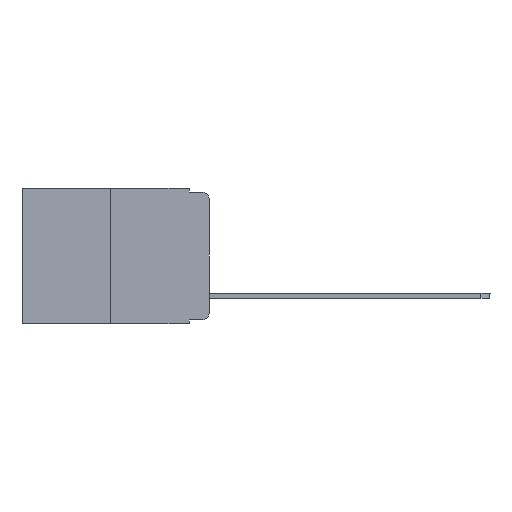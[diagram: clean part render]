
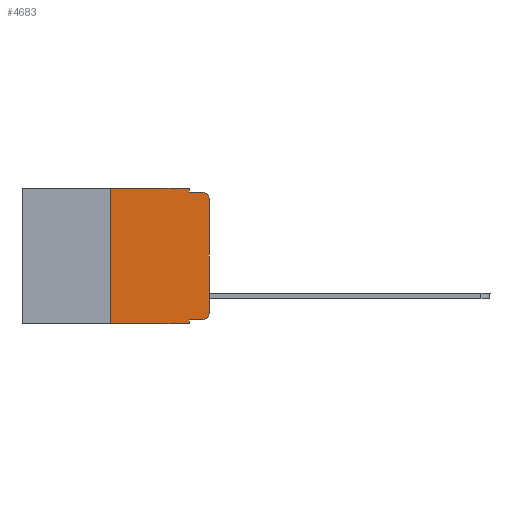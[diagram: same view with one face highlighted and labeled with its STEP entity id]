
A CAD part, left-side view. The second image highlights one B-rep face of the part: STEP entity #4683.
In plain terms, the highlighted planar face has unit normal (-1, 0, 0).
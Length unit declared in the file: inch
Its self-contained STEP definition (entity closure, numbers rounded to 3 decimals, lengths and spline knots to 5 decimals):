
#188 = CARTESIAN_POINT ( 'NONE',  ( 0., 0., -0.03 ) ) ;
#470 = EDGE_CURVE ( 'NONE', #12312, #9007, #893, .T. ) ;
#848 = DIRECTION ( 'NONE',  ( 0., 0., -1. ) ) ;
#893 = LINE ( 'NONE', #14707, #12993 ) ;
#906 = DIRECTION ( 'NONE',  ( 0., 0., -1. ) ) ;
#1216 = VERTEX_POINT ( 'NONE', #9771 ) ;
#1323 = EDGE_CURVE ( 'NONE', #9047, #8708, #15082, .T. ) ;
#1402 = LINE ( 'NONE', #6682, #8068 ) ;
#1823 = DIRECTION ( 'NONE',  ( 0., -1., 0. ) ) ;
#2102 = VERTEX_POINT ( 'NONE', #5458 ) ;
#2106 = LINE ( 'NONE', #5754, #11405 ) ;
#2135 = EDGE_CURVE ( 'NONE', #2807, #11199, #7051, .T. ) ;
#2204 = LINE ( 'NONE', #2938, #13914 ) ;
#2452 = CARTESIAN_POINT ( 'NONE',  ( 0., 0.051, 0. ) ) ;
#2599 = EDGE_CURVE ( 'NONE', #9047, #2102, #2204, .T. ) ;
#2780 = ORIENTED_EDGE ( 'NONE', *, *, #1323, .F. ) ;
#2807 = VERTEX_POINT ( 'NONE', #4422 ) ;
#2938 = CARTESIAN_POINT ( 'NONE',  ( 0., 0.051, -0.333 ) ) ;
#3045 = DIRECTION ( 'NONE',  ( 0., -1., 0. ) ) ;
#3590 = LINE ( 'NONE', #7169, #11811 ) ;
#4154 = CARTESIAN_POINT ( 'NONE',  ( 0., 0.051, 0. ) ) ;
#4384 = CARTESIAN_POINT ( 'NONE',  ( 0., 0.051, -0.343 ) ) ;
#4396 = DIRECTION ( 'NONE',  ( 0., 0., 1. ) ) ;
#4422 = CARTESIAN_POINT ( 'NONE',  ( 0., 0., -0.313 ) ) ;
#4469 = ORIENTED_EDGE ( 'NONE', *, *, #470, .F. ) ;
#4472 = CARTESIAN_POINT ( 'NONE',  ( 0., 0.02, -0.313 ) ) ;
#4581 = DIRECTION ( 'NONE',  ( -1., 0., 0. ) ) ;
#4683 = ADVANCED_FACE ( 'NONE', ( #11479 ), #10217, .F. ) ;
#5392 = CARTESIAN_POINT ( 'NONE',  ( 0., 0.25, -0.343 ) ) ;
#5458 = CARTESIAN_POINT ( 'NONE',  ( 0., 0.02, -0.333 ) ) ;
#5754 = CARTESIAN_POINT ( 'NONE',  ( 0., 0.051, -0.01 ) ) ;
#6182 = ORIENTED_EDGE ( 'NONE', *, *, #2135, .T. ) ;
#6511 = DIRECTION ( 'NONE',  ( 0., -1., 0. ) ) ;
#6682 = CARTESIAN_POINT ( 'NONE',  ( 0., 0.473, -0.343 ) ) ;
#6736 = ORIENTED_EDGE ( 'NONE', *, *, #12815, .F. ) ;
#6756 = CARTESIAN_POINT ( 'NONE',  ( 0., 0.051, -0.01 ) ) ;
#6867 = EDGE_CURVE ( 'NONE', #10242, #12312, #3590, .T. ) ;
#6870 = CARTESIAN_POINT ( 'NONE',  ( 0., 0.051, 0. ) ) ;
#7051 = LINE ( 'NONE', #11347, #10215 ) ;
#7169 = CARTESIAN_POINT ( 'NONE',  ( 0., 0.25, 0. ) ) ;
#7179 = DIRECTION ( 'NONE',  ( 0., 0., -1. ) ) ;
#7481 = VERTEX_POINT ( 'NONE', #6756 ) ;
#7965 = EDGE_CURVE ( 'NONE', #10242, #8708, #1402, .T. ) ;
#8017 = ORIENTED_EDGE ( 'NONE', *, *, #14210, .T. ) ;
#8068 = VECTOR ( 'NONE', #1823, 39.37008 ) ;
#8161 = AXIS2_PLACEMENT_3D ( 'NONE', #12897, #15297, #10874 ) ;
#8309 = CARTESIAN_POINT ( 'NONE',  ( 0., 0.25, 0. ) ) ;
#8338 = VECTOR ( 'NONE', #11307, 39.37008 ) ;
#8708 = VERTEX_POINT ( 'NONE', #4384 ) ;
#9007 = VERTEX_POINT ( 'NONE', #6870 ) ;
#9041 = EDGE_LOOP ( 'NONE', ( #6182, #8017, #6736, #10546, #4469, #13169, #9443, #2780, #13360, #9932 ) ) ;
#9047 = VERTEX_POINT ( 'NONE', #10814 ) ;
#9443 = ORIENTED_EDGE ( 'NONE', *, *, #7965, .T. ) ;
#9665 = CIRCLE ( 'NONE', #8161, 0.02 ) ;
#9771 = CARTESIAN_POINT ( 'NONE',  ( 0., 0.02, -0.01 ) ) ;
#9791 = AXIS2_PLACEMENT_3D ( 'NONE', #13889, #10166, #848 ) ;
#9932 = ORIENTED_EDGE ( 'NONE', *, *, #11006, .T. ) ;
#10166 = DIRECTION ( 'NONE',  ( 1., 0., 0. ) ) ;
#10215 = VECTOR ( 'NONE', #4396, 39.37008 ) ;
#10217 = PLANE ( 'NONE',  #9791 ) ;
#10242 = VERTEX_POINT ( 'NONE', #5392 ) ;
#10523 = AXIS2_PLACEMENT_3D ( 'NONE', #4472, #4581, #906 ) ;
#10546 = ORIENTED_EDGE ( 'NONE', *, *, #11414, .F. ) ;
#10551 = DIRECTION ( 'NONE',  ( 0., -1., 0. ) ) ;
#10756 = DIRECTION ( 'NONE',  ( 0., 0., 1. ) ) ;
#10814 = CARTESIAN_POINT ( 'NONE',  ( 0., 0.051, -0.333 ) ) ;
#10874 = DIRECTION ( 'NONE',  ( 0., 0., -1. ) ) ;
#11006 = EDGE_CURVE ( 'NONE', #2102, #2807, #15427, .T. ) ;
#11199 = VERTEX_POINT ( 'NONE', #188 ) ;
#11307 = DIRECTION ( 'NONE',  ( 0., 0., -1. ) ) ;
#11347 = CARTESIAN_POINT ( 'NONE',  ( 0., 0., 0. ) ) ;
#11405 = VECTOR ( 'NONE', #10551, 39.37008 ) ;
#11414 = EDGE_CURVE ( 'NONE', #9007, #7481, #13164, .T. ) ;
#11479 = FACE_OUTER_BOUND ( 'NONE', #9041, .T. ) ;
#11811 = VECTOR ( 'NONE', #10756, 39.37008 ) ;
#12312 = VERTEX_POINT ( 'NONE', #8309 ) ;
#12815 = EDGE_CURVE ( 'NONE', #7481, #1216, #2106, .T. ) ;
#12897 = CARTESIAN_POINT ( 'NONE',  ( 0., 0.02, -0.03 ) ) ;
#12993 = VECTOR ( 'NONE', #6511, 39.37008 ) ;
#13164 = LINE ( 'NONE', #4154, #8338 ) ;
#13169 = ORIENTED_EDGE ( 'NONE', *, *, #6867, .F. ) ;
#13360 = ORIENTED_EDGE ( 'NONE', *, *, #2599, .T. ) ;
#13889 = CARTESIAN_POINT ( 'NONE',  ( 0., 0.473, 0. ) ) ;
#13914 = VECTOR ( 'NONE', #3045, 39.37008 ) ;
#14210 = EDGE_CURVE ( 'NONE', #11199, #1216, #9665, .T. ) ;
#14707 = CARTESIAN_POINT ( 'NONE',  ( 0., 0.473, 0. ) ) ;
#15082 = LINE ( 'NONE', #2452, #15271 ) ;
#15271 = VECTOR ( 'NONE', #7179, 39.37008 ) ;
#15297 = DIRECTION ( 'NONE',  ( -1., 0., 0. ) ) ;
#15427 = CIRCLE ( 'NONE', #10523, 0.02 ) ;
